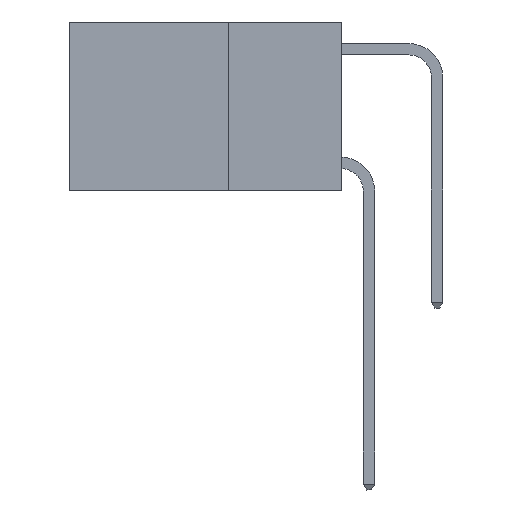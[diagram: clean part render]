
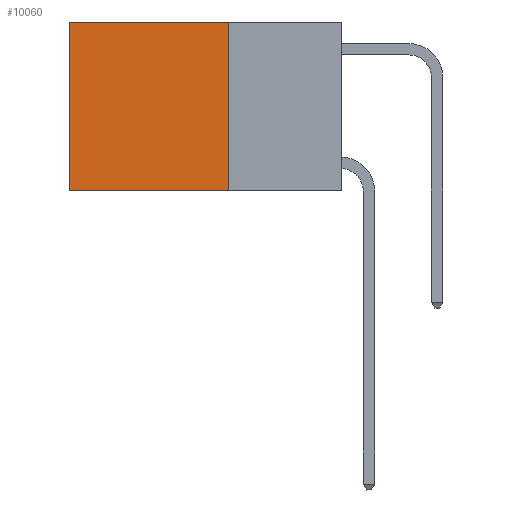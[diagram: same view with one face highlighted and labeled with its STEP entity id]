
A CAD part, left-side view. The second image highlights one B-rep face of the part: STEP entity #10060.
In plain terms, the highlighted planar face has unit normal (-1, 0, 0).
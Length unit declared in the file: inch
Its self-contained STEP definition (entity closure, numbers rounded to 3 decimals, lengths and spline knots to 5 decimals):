
#40 = DIRECTION ( 'NONE',  ( 0., 0., -1. ) ) ;
#215 = ORIENTED_EDGE ( 'NONE', *, *, #13671, .T. ) ;
#283 = CARTESIAN_POINT ( 'NONE',  ( 0.2625, 0.25, 0. ) ) ;
#392 = AXIS2_PLACEMENT_3D ( 'NONE', #4038, #7269, #2938 ) ;
#410 = VERTEX_POINT ( 'NONE', #4576 ) ;
#930 = VERTEX_POINT ( 'NONE', #1410 ) ;
#1160 = CARTESIAN_POINT ( 'NONE',  ( 0.2625, 0.6, 0. ) ) ;
#1191 = LINE ( 'NONE', #5489, #10237 ) ;
#1410 = CARTESIAN_POINT ( 'NONE',  ( 0.2625, 0.6, 0. ) ) ;
#1550 = VERTEX_POINT ( 'NONE', #9033 ) ;
#2457 = ORIENTED_EDGE ( 'NONE', *, *, #12555, .T. ) ;
#2938 = DIRECTION ( 'NONE',  ( 0., 0., -1. ) ) ;
#3006 = LINE ( 'NONE', #1160, #10479 ) ;
#4027 = DIRECTION ( 'NONE',  ( 0., 1., 0. ) ) ;
#4038 = CARTESIAN_POINT ( 'NONE',  ( 0.2625, 0.25, 0. ) ) ;
#4043 = EDGE_CURVE ( 'NONE', #410, #1550, #10379, .T. ) ;
#4539 = DIRECTION ( 'NONE',  ( 0., 0., -1. ) ) ;
#4576 = CARTESIAN_POINT ( 'NONE',  ( 0.2625, 0.25, -0.37 ) ) ;
#5443 = EDGE_CURVE ( 'NONE', #8728, #410, #9807, .T. ) ;
#5489 = CARTESIAN_POINT ( 'NONE',  ( 0.2625, 0.25, 0. ) ) ;
#7269 = DIRECTION ( 'NONE',  ( 1., 0., 0. ) ) ;
#7715 = DIRECTION ( 'NONE',  ( 0., 1., 0. ) ) ;
#7758 = VECTOR ( 'NONE', #4027, 39.37008 ) ;
#7810 = ORIENTED_EDGE ( 'NONE', *, *, #4043, .F. ) ;
#8713 = ORIENTED_EDGE ( 'NONE', *, *, #5443, .F. ) ;
#8728 = VERTEX_POINT ( 'NONE', #9069 ) ;
#9033 = CARTESIAN_POINT ( 'NONE',  ( 0.2625, 0.6, -0.37 ) ) ;
#9069 = CARTESIAN_POINT ( 'NONE',  ( 0.2625, 0.25, 0. ) ) ;
#9807 = LINE ( 'NONE', #283, #12007 ) ;
#10060 = ADVANCED_FACE ( 'NONE', ( #13547 ), #12427, .F. ) ;
#10237 = VECTOR ( 'NONE', #7715, 39.37008 ) ;
#10379 = LINE ( 'NONE', #13649, #7758 ) ;
#10479 = VECTOR ( 'NONE', #40, 39.37008 ) ;
#11140 = EDGE_LOOP ( 'NONE', ( #215, #7810, #8713, #2457 ) ) ;
#12007 = VECTOR ( 'NONE', #4539, 39.37008 ) ;
#12427 = PLANE ( 'NONE',  #392 ) ;
#12555 = EDGE_CURVE ( 'NONE', #8728, #930, #1191, .T. ) ;
#13547 = FACE_OUTER_BOUND ( 'NONE', #11140, .T. ) ;
#13649 = CARTESIAN_POINT ( 'NONE',  ( 0.2625, 0.25, -0.37 ) ) ;
#13671 = EDGE_CURVE ( 'NONE', #930, #1550, #3006, .T. ) ;
